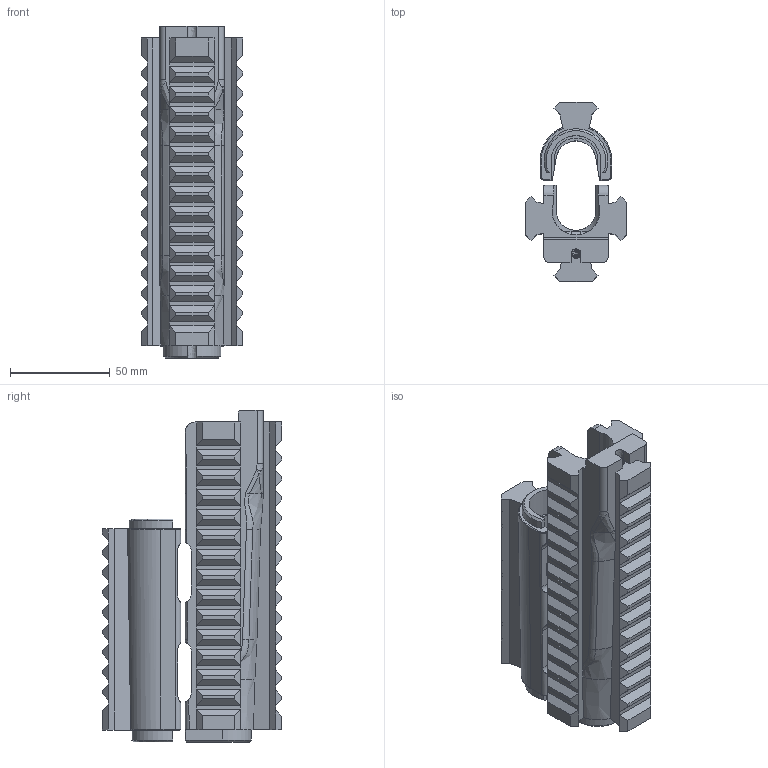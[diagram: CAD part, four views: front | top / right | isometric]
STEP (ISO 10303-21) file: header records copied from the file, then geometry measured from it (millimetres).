
FILE_DESCRIPTION(/* description */ (''),/* implementation_level */ '2;1');
FILE_NAME(/* name */ 'AK FOREGRIPS.stp',/* time_stamp */ '2021-03-21T13:21:00+01:00',/* author */ (''),/* organization */ (''),/* preprocessor_version */ 'ST-DEVELOPER v15.2',/* originating_system */ 'Autodesk Translator Framework v2.0.0.5431',/* authorisation */ '');
FILE_SCHEMA (('AUTOMOTIVE_DESIGN { 1 0 10303 214 3 1 1 }'));
Length unit declared in the file: centimetre
Products named in the file (1): AKM RAILED GRIPS
Bounding box: 50.9 x 89.77 x 166.3 mm (x, y, z)
Volume: 225619.1 mm3; surface area: 66119.8 mm2
Topology: 2 solids, 2 shells, 527 faces, 1341 edges, 814 vertices
Faces by surface type: plane 415, cylinder 61, bspline 43, cone 4, torus 4
Full cylindrical faces by diameter (mm): 7 x1
Entity records: 21774 total; most frequent: CARTESIAN_POINT 9522, ORIENTED_EDGE 2670, DIRECTION 2298, EDGE_CURVE 1335, LINE 1058, VECTOR 1058, VERTEX_POINT 812, AXIS2_PLACEMENT_3D 620
